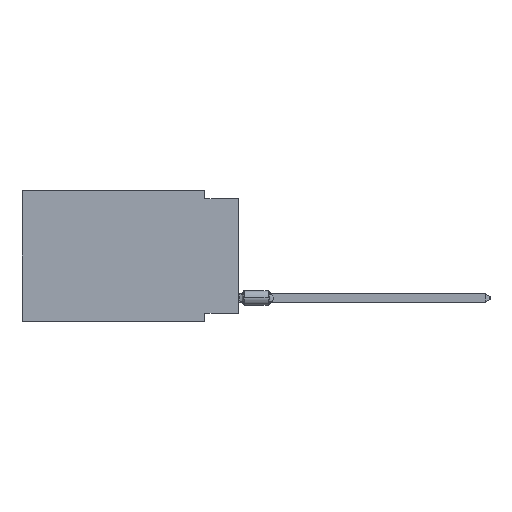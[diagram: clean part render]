
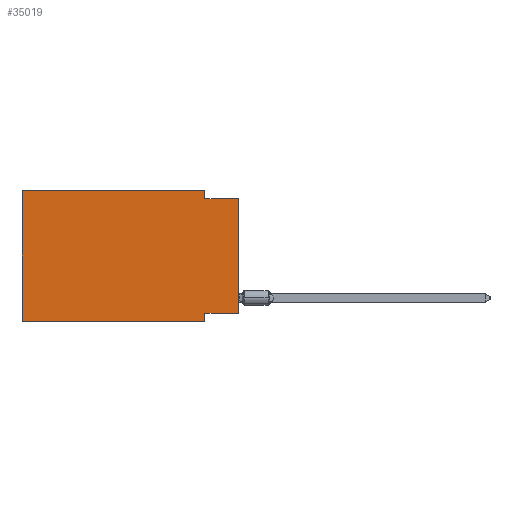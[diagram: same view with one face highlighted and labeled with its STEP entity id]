
A CAD part, left-side view. The second image highlights one B-rep face of the part: STEP entity #35019.
In plain terms, the highlighted planar face has unit normal (-1, 0, 0).
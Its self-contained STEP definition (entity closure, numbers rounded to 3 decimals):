
#444 = ORIENTED_EDGE ( 'NONE', *, *, #14474, .F. ) ;
#1179 = DIRECTION ( 'NONE',  ( 0., 1., 0. ) ) ;
#2052 = LINE ( 'NONE', #36390, #11266 ) ;
#2646 = CARTESIAN_POINT ( 'NONE',  ( 0., 16.383, 0. ) ) ;
#3480 = ORIENTED_EDGE ( 'NONE', *, *, #9946, .T. ) ;
#4047 = DIRECTION ( 'NONE',  ( 0., -1., 0. ) ) ;
#4833 = VERTEX_POINT ( 'NONE', #38548 ) ;
#5470 = CARTESIAN_POINT ( 'NONE',  ( 0., 2.54, -9.906 ) ) ;
#6050 = VECTOR ( 'NONE', #39008, 1000. ) ;
#6270 = CARTESIAN_POINT ( 'NONE',  ( 0., 16.383, 0. ) ) ;
#6445 = CARTESIAN_POINT ( 'NONE',  ( 0., 16.383, -9.906 ) ) ;
#6462 = LINE ( 'NONE', #6270, #31976 ) ;
#7233 = VERTEX_POINT ( 'NONE', #7530 ) ;
#7353 = LINE ( 'NONE', #16296, #26895 ) ;
#7530 = CARTESIAN_POINT ( 'NONE',  ( 0., 2.54, -0.635 ) ) ;
#9448 = CARTESIAN_POINT ( 'NONE',  ( 0., 2.54, 0. ) ) ;
#9946 = EDGE_CURVE ( 'NONE', #10607, #4833, #2052, .T. ) ;
#10231 = CARTESIAN_POINT ( 'NONE',  ( 0., 2.54, 0. ) ) ;
#10235 = EDGE_CURVE ( 'NONE', #7233, #27869, #19075, .T. ) ;
#10339 = EDGE_LOOP ( 'NONE', ( #19076, #39445, #444, #37913, #27676, #3480, #31909, #13667 ) ) ;
#10607 = VERTEX_POINT ( 'NONE', #6445 ) ;
#10696 = CARTESIAN_POINT ( 'NONE',  ( 0., 0., -9.271 ) ) ;
#10968 = DIRECTION ( 'NONE',  ( 0., -1., 0. ) ) ;
#11266 = VECTOR ( 'NONE', #10968, 1000. ) ;
#11970 = DIRECTION ( 'NONE',  ( 1., 0., 0. ) ) ;
#13667 = ORIENTED_EDGE ( 'NONE', *, *, #24725, .F. ) ;
#13678 = LINE ( 'NONE', #10231, #33519 ) ;
#14020 = CARTESIAN_POINT ( 'NONE',  ( 0., 0., -0.635 ) ) ;
#14474 = EDGE_CURVE ( 'NONE', #17020, #7233, #13678, .T. ) ;
#14849 = CARTESIAN_POINT ( 'NONE',  ( 0., 0., -9.271 ) ) ;
#15835 = CARTESIAN_POINT ( 'NONE',  ( 0., 0., -0.635 ) ) ;
#16296 = CARTESIAN_POINT ( 'NONE',  ( 0., 0., 0. ) ) ;
#17020 = VERTEX_POINT ( 'NONE', #9448 ) ;
#17468 = DIRECTION ( 'NONE',  ( 0., 0., -1. ) ) ;
#18836 = DIRECTION ( 'NONE',  ( 0., -1., 0. ) ) ;
#19075 = LINE ( 'NONE', #15835, #22093 ) ;
#19076 = ORIENTED_EDGE ( 'NONE', *, *, #26564, .T. ) ;
#21174 = VERTEX_POINT ( 'NONE', #39419 ) ;
#22093 = VECTOR ( 'NONE', #4047, 1000. ) ;
#22119 = EDGE_CURVE ( 'NONE', #21174, #4833, #36164, .T. ) ;
#22645 = DIRECTION ( 'NONE',  ( 0., 0., -1. ) ) ;
#23350 = EDGE_CURVE ( 'NONE', #27912, #17020, #6462, .T. ) ;
#24725 = EDGE_CURVE ( 'NONE', #30484, #21174, #31468, .T. ) ;
#26564 = EDGE_CURVE ( 'NONE', #30484, #27869, #7353, .T. ) ;
#26710 = CARTESIAN_POINT ( 'NONE',  ( 0., 16.383, 0. ) ) ;
#26895 = VECTOR ( 'NONE', #29101, 1000. ) ;
#27676 = ORIENTED_EDGE ( 'NONE', *, *, #33914, .F. ) ;
#27868 = VECTOR ( 'NONE', #36263, 1000. ) ;
#27869 = VERTEX_POINT ( 'NONE', #14020 ) ;
#27912 = VERTEX_POINT ( 'NONE', #29470 ) ;
#29101 = DIRECTION ( 'NONE',  ( 0., 0., 1. ) ) ;
#29470 = CARTESIAN_POINT ( 'NONE',  ( 0., 16.383, 0. ) ) ;
#30482 = FACE_OUTER_BOUND ( 'NONE', #10339, .T. ) ;
#30484 = VERTEX_POINT ( 'NONE', #14849 ) ;
#31468 = LINE ( 'NONE', #10696, #36627 ) ;
#31909 = ORIENTED_EDGE ( 'NONE', *, *, #22119, .F. ) ;
#31976 = VECTOR ( 'NONE', #18836, 1000. ) ;
#33519 = VECTOR ( 'NONE', #22645, 1000. ) ;
#33772 = AXIS2_PLACEMENT_3D ( 'NONE', #2646, #11970, #17468 ) ;
#33914 = EDGE_CURVE ( 'NONE', #10607, #27912, #39525, .T. ) ;
#35019 = ADVANCED_FACE ( 'NONE', ( #30482 ), #36190, .F. ) ;
#36164 = LINE ( 'NONE', #5470, #6050 ) ;
#36190 = PLANE ( 'NONE',  #33772 ) ;
#36263 = DIRECTION ( 'NONE',  ( 0., 0., 1. ) ) ;
#36390 = CARTESIAN_POINT ( 'NONE',  ( 0., 16.383, -9.906 ) ) ;
#36627 = VECTOR ( 'NONE', #1179, 1000. ) ;
#37913 = ORIENTED_EDGE ( 'NONE', *, *, #23350, .F. ) ;
#38548 = CARTESIAN_POINT ( 'NONE',  ( 0., 2.54, -9.906 ) ) ;
#39008 = DIRECTION ( 'NONE',  ( 0., 0., -1. ) ) ;
#39419 = CARTESIAN_POINT ( 'NONE',  ( 0., 2.54, -9.271 ) ) ;
#39445 = ORIENTED_EDGE ( 'NONE', *, *, #10235, .F. ) ;
#39525 = LINE ( 'NONE', #26710, #27868 ) ;
